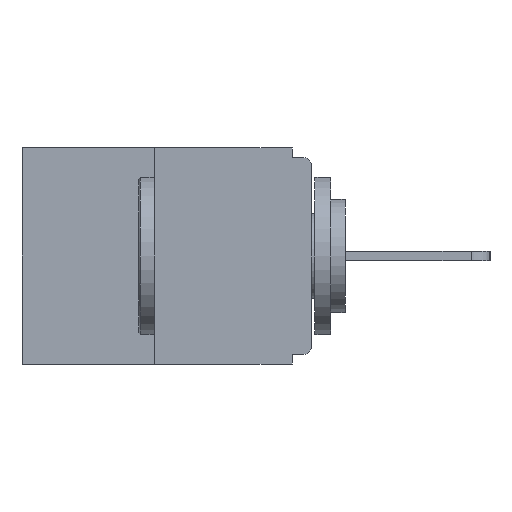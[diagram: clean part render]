
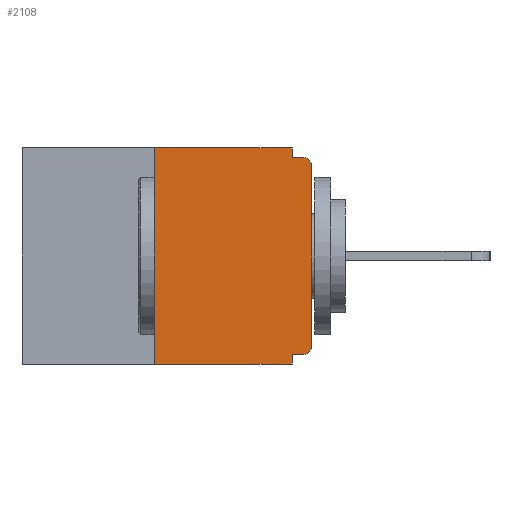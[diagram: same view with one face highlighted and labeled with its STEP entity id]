
A CAD part, left-side view. The second image highlights one B-rep face of the part: STEP entity #2108.
In plain terms, the highlighted planar face has unit normal (-1, 0, 0).
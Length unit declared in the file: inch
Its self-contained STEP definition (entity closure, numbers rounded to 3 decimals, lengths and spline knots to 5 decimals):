
#296 = CIRCLE ( 'NONE', #4165, 0.015 ) ;
#330 = VERTEX_POINT ( 'NONE', #10038 ) ;
#580 = CARTESIAN_POINT ( 'NONE',  ( 0., 0.46, 0. ) ) ;
#772 = CIRCLE ( 'NONE', #16095, 0.015 ) ;
#924 = ORIENTED_EDGE ( 'NONE', *, *, #11124, .T. ) ;
#1372 = VERTEX_POINT ( 'NONE', #3596 ) ;
#1406 = EDGE_CURVE ( 'NONE', #15183, #15429, #14429, .T. ) ;
#1475 = DIRECTION ( 'NONE',  ( 0., -1., 0. ) ) ;
#1528 = EDGE_CURVE ( 'NONE', #1893, #1372, #13240, .T. ) ;
#1623 = DIRECTION ( 'NONE',  ( 0., 0., -1. ) ) ;
#1842 = DIRECTION ( 'NONE',  ( -1., 0., 0. ) ) ;
#1893 = VERTEX_POINT ( 'NONE', #8650 ) ;
#1909 = ORIENTED_EDGE ( 'NONE', *, *, #1406, .F. ) ;
#2043 = CARTESIAN_POINT ( 'NONE',  ( 0., 0.031, -0.328 ) ) ;
#2108 = ADVANCED_FACE ( 'NONE', ( #12074 ), #5633, .F. ) ;
#2116 = CARTESIAN_POINT ( 'NONE',  ( 0., 0.031, -0.343 ) ) ;
#2212 = EDGE_CURVE ( 'NONE', #15429, #330, #15963, .T. ) ;
#2395 = CARTESIAN_POINT ( 'NONE',  ( 0., 0.015, -0.328 ) ) ;
#2582 = CARTESIAN_POINT ( 'NONE',  ( 0., 0., -0.03 ) ) ;
#2915 = DIRECTION ( 'NONE',  ( 0., -1., 0. ) ) ;
#3093 = CARTESIAN_POINT ( 'NONE',  ( 0., 0.031, 0. ) ) ;
#3125 = DIRECTION ( 'NONE',  ( 0., 0., 1. ) ) ;
#3460 = CARTESIAN_POINT ( 'NONE',  ( 0., 0.25, -0.343 ) ) ;
#3596 = CARTESIAN_POINT ( 'NONE',  ( 0., 0.015, -0.015 ) ) ;
#4036 = ORIENTED_EDGE ( 'NONE', *, *, #5797, .F. ) ;
#4083 = VECTOR ( 'NONE', #3125, 39.37008 ) ;
#4165 = AXIS2_PLACEMENT_3D ( 'NONE', #10612, #1842, #1623 ) ;
#4220 = EDGE_CURVE ( 'NONE', #15183, #5190, #772, .T. ) ;
#4418 = DIRECTION ( 'NONE',  ( 0., 0., -1. ) ) ;
#4638 = CARTESIAN_POINT ( 'NONE',  ( 0., 0., 0. ) ) ;
#5000 = CARTESIAN_POINT ( 'NONE',  ( 0., 0., -0.313 ) ) ;
#5190 = VERTEX_POINT ( 'NONE', #5000 ) ;
#5545 = ORIENTED_EDGE ( 'NONE', *, *, #11544, .F. ) ;
#5561 = VERTEX_POINT ( 'NONE', #2582 ) ;
#5633 = PLANE ( 'NONE',  #7786 ) ;
#5797 = EDGE_CURVE ( 'NONE', #6110, #6462, #9795, .T. ) ;
#5819 = ORIENTED_EDGE ( 'NONE', *, *, #13706, .F. ) ;
#6011 = EDGE_CURVE ( 'NONE', #5190, #5561, #16070, .T. ) ;
#6110 = VERTEX_POINT ( 'NONE', #3460 ) ;
#6462 = VERTEX_POINT ( 'NONE', #13230 ) ;
#6913 = ORIENTED_EDGE ( 'NONE', *, *, #7702, .T. ) ;
#7016 = VECTOR ( 'NONE', #8255, 39.37008 ) ;
#7427 = LINE ( 'NONE', #10884, #7016 ) ;
#7543 = ORIENTED_EDGE ( 'NONE', *, *, #1528, .F. ) ;
#7544 = ORIENTED_EDGE ( 'NONE', *, *, #6011, .T. ) ;
#7572 = CARTESIAN_POINT ( 'NONE',  ( 0., 0., -0.328 ) ) ;
#7702 = EDGE_CURVE ( 'NONE', #6110, #330, #13639, .T. ) ;
#7779 = CARTESIAN_POINT ( 'NONE',  ( 0., 0., -0.015 ) ) ;
#7786 = AXIS2_PLACEMENT_3D ( 'NONE', #580, #8087, #9397 ) ;
#8087 = DIRECTION ( 'NONE',  ( 1., 0., 0. ) ) ;
#8255 = DIRECTION ( 'NONE',  ( 0., 0., -1. ) ) ;
#8400 = ORIENTED_EDGE ( 'NONE', *, *, #4220, .T. ) ;
#8650 = CARTESIAN_POINT ( 'NONE',  ( 0., 0.031, -0.015 ) ) ;
#8944 = VECTOR ( 'NONE', #2915, 39.37008 ) ;
#9397 = DIRECTION ( 'NONE',  ( 0., 0., -1. ) ) ;
#9795 = LINE ( 'NONE', #13992, #4083 ) ;
#9951 = LINE ( 'NONE', #12745, #14040 ) ;
#10038 = CARTESIAN_POINT ( 'NONE',  ( 0., 0.031, -0.343 ) ) ;
#10039 = CARTESIAN_POINT ( 'NONE',  ( 0., 0.46, -0.343 ) ) ;
#10612 = CARTESIAN_POINT ( 'NONE',  ( 0., 0.015, -0.03 ) ) ;
#10884 = CARTESIAN_POINT ( 'NONE',  ( 0., 0.031, 0. ) ) ;
#11064 = DIRECTION ( 'NONE',  ( 0., 0., -1. ) ) ;
#11124 = EDGE_CURVE ( 'NONE', #5561, #1372, #296, .T. ) ;
#11318 = DIRECTION ( 'NONE',  ( 0., -1., 0. ) ) ;
#11460 = DIRECTION ( 'NONE',  ( 0., 1., 0. ) ) ;
#11544 = EDGE_CURVE ( 'NONE', #12994, #1893, #7427, .T. ) ;
#11929 = DIRECTION ( 'NONE',  ( -1., 0., 0. ) ) ;
#12074 = FACE_OUTER_BOUND ( 'NONE', #14432, .T. ) ;
#12708 = VECTOR ( 'NONE', #15753, 39.37008 ) ;
#12745 = CARTESIAN_POINT ( 'NONE',  ( 0., 0.46, 0. ) ) ;
#12994 = VERTEX_POINT ( 'NONE', #3093 ) ;
#13230 = CARTESIAN_POINT ( 'NONE',  ( 0., 0.25, 0. ) ) ;
#13240 = LINE ( 'NONE', #7779, #8944 ) ;
#13327 = CARTESIAN_POINT ( 'NONE',  ( 0., 0.015, -0.313 ) ) ;
#13639 = LINE ( 'NONE', #10039, #14811 ) ;
#13706 = EDGE_CURVE ( 'NONE', #6462, #12994, #9951, .T. ) ;
#13992 = CARTESIAN_POINT ( 'NONE',  ( 0., 0.25, 0. ) ) ;
#14040 = VECTOR ( 'NONE', #1475, 39.37008 ) ;
#14429 = LINE ( 'NONE', #7572, #15019 ) ;
#14432 = EDGE_LOOP ( 'NONE', ( #5819, #4036, #6913, #15452, #1909, #8400, #7544, #924, #7543, #5545 ) ) ;
#14811 = VECTOR ( 'NONE', #11318, 39.37008 ) ;
#15019 = VECTOR ( 'NONE', #11460, 39.37008 ) ;
#15183 = VERTEX_POINT ( 'NONE', #2395 ) ;
#15429 = VERTEX_POINT ( 'NONE', #2043 ) ;
#15452 = ORIENTED_EDGE ( 'NONE', *, *, #2212, .F. ) ;
#15753 = DIRECTION ( 'NONE',  ( 0., 0., 1. ) ) ;
#15963 = LINE ( 'NONE', #2116, #16175 ) ;
#16070 = LINE ( 'NONE', #4638, #12708 ) ;
#16095 = AXIS2_PLACEMENT_3D ( 'NONE', #13327, #11929, #4418 ) ;
#16175 = VECTOR ( 'NONE', #11064, 39.37008 ) ;
